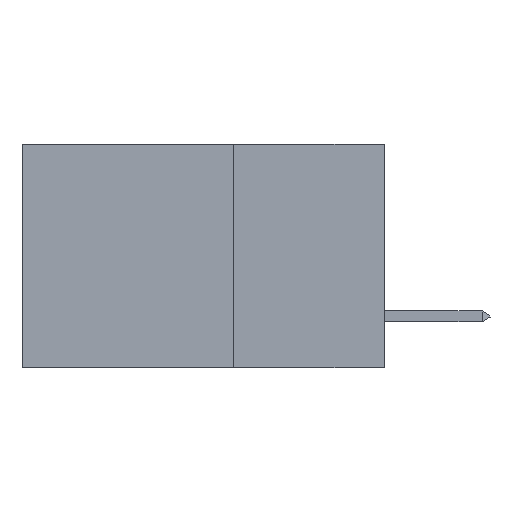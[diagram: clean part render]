
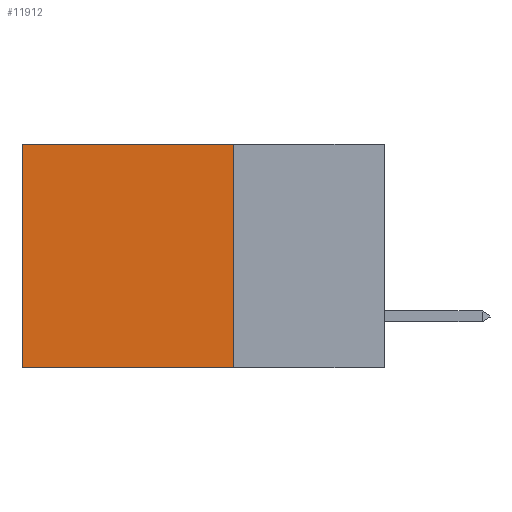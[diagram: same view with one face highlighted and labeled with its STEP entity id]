
A CAD part, left-side view. The second image highlights one B-rep face of the part: STEP entity #11912.
In plain terms, the highlighted planar face has unit normal (-1, 0, 0).
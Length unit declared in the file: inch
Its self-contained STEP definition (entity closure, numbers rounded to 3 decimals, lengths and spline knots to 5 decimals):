
#105 = VERTEX_POINT ( 'NONE', #4023 ) ;
#658 = EDGE_CURVE ( 'NONE', #9398, #10894, #5657, .T. ) ;
#699 = EDGE_CURVE ( 'NONE', #105, #9398, #6534, .T. ) ;
#710 = VERTEX_POINT ( 'NONE', #8863 ) ;
#1538 = LINE ( 'NONE', #3732, #9543 ) ;
#2034 = DIRECTION ( 'NONE',  ( 0., 1., 0. ) ) ;
#2689 = EDGE_CURVE ( 'NONE', #105, #710, #1538, .T. ) ;
#2835 = CARTESIAN_POINT ( 'NONE',  ( 0.2875, 0.6, -0.37 ) ) ;
#2934 = ORIENTED_EDGE ( 'NONE', *, *, #658, .T. ) ;
#3732 = CARTESIAN_POINT ( 'NONE',  ( 0.2875, 0.25, 0. ) ) ;
#4023 = CARTESIAN_POINT ( 'NONE',  ( 0.2875, 0.25, 0. ) ) ;
#4205 = ORIENTED_EDGE ( 'NONE', *, *, #2689, .F. ) ;
#4324 = DIRECTION ( 'NONE',  ( 1., 0., 0. ) ) ;
#5173 = ORIENTED_EDGE ( 'NONE', *, *, #699, .T. ) ;
#5350 = DIRECTION ( 'NONE',  ( 0., 0., -1. ) ) ;
#5657 = LINE ( 'NONE', #11585, #9117 ) ;
#6131 = EDGE_LOOP ( 'NONE', ( #2934, #9947, #4205, #5173 ) ) ;
#6534 = LINE ( 'NONE', #7980, #10676 ) ;
#7137 = CARTESIAN_POINT ( 'NONE',  ( 0.2875, 0.25, 0. ) ) ;
#7814 = CARTESIAN_POINT ( 'NONE',  ( 0.2875, 0.25, -0.37 ) ) ;
#7980 = CARTESIAN_POINT ( 'NONE',  ( 0.2875, 0.25, 0. ) ) ;
#8009 = FACE_OUTER_BOUND ( 'NONE', #6131, .T. ) ;
#8863 = CARTESIAN_POINT ( 'NONE',  ( 0.2875, 0.25, -0.37 ) ) ;
#9044 = PLANE ( 'NONE',  #10669 ) ;
#9117 = VECTOR ( 'NONE', #9582, 39.37008 ) ;
#9398 = VERTEX_POINT ( 'NONE', #11943 ) ;
#9543 = VECTOR ( 'NONE', #10627, 39.37008 ) ;
#9582 = DIRECTION ( 'NONE',  ( 0., 0., -1. ) ) ;
#9805 = DIRECTION ( 'NONE',  ( 0., 1., 0. ) ) ;
#9947 = ORIENTED_EDGE ( 'NONE', *, *, #12210, .F. ) ;
#10573 = LINE ( 'NONE', #7814, #11773 ) ;
#10627 = DIRECTION ( 'NONE',  ( 0., 0., -1. ) ) ;
#10669 = AXIS2_PLACEMENT_3D ( 'NONE', #7137, #4324, #5350 ) ;
#10676 = VECTOR ( 'NONE', #9805, 39.37008 ) ;
#10894 = VERTEX_POINT ( 'NONE', #2835 ) ;
#11585 = CARTESIAN_POINT ( 'NONE',  ( 0.2875, 0.6, 0. ) ) ;
#11773 = VECTOR ( 'NONE', #2034, 39.37008 ) ;
#11912 = ADVANCED_FACE ( 'NONE', ( #8009 ), #9044, .F. ) ;
#11943 = CARTESIAN_POINT ( 'NONE',  ( 0.2875, 0.6, 0. ) ) ;
#12210 = EDGE_CURVE ( 'NONE', #710, #10894, #10573, .T. ) ;
